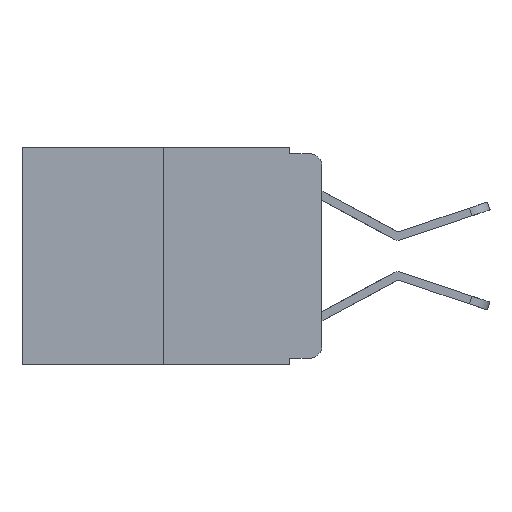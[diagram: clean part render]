
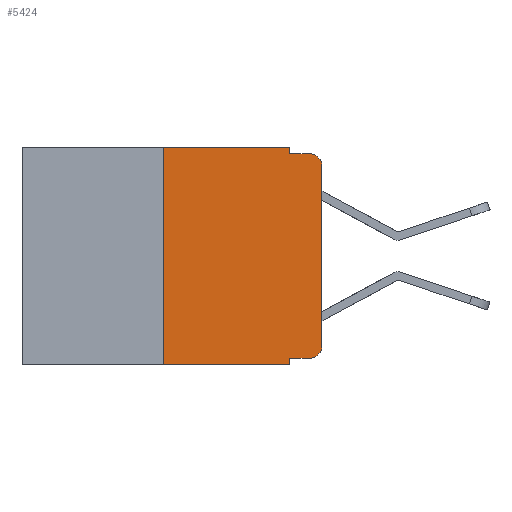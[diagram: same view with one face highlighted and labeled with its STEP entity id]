
A CAD part, left-side view. The second image highlights one B-rep face of the part: STEP entity #5424.
In plain terms, the highlighted planar face has unit normal (-1, 0, 0).
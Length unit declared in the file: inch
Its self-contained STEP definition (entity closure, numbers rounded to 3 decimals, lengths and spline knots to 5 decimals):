
#252 = CIRCLE ( 'NONE', #13759, 0.02 ) ;
#501 = DIRECTION ( 'NONE',  ( -1., 0., 0. ) ) ;
#651 = EDGE_LOOP ( 'NONE', ( #2425, #10456, #5234, #5033, #9141, #5659, #2915, #13785, #4641, #11686 ) ) ;
#1095 = PLANE ( 'NONE',  #2298 ) ;
#1150 = VERTEX_POINT ( 'NONE', #14654 ) ;
#1448 = DIRECTION ( 'NONE',  ( 0., 0., -1. ) ) ;
#1543 = EDGE_CURVE ( 'NONE', #1150, #5483, #14541, .T. ) ;
#2195 = EDGE_CURVE ( 'NONE', #3941, #1150, #7208, .T. ) ;
#2298 = AXIS2_PLACEMENT_3D ( 'NONE', #10191, #10025, #14856 ) ;
#2425 = ORIENTED_EDGE ( 'NONE', *, *, #8944, .T. ) ;
#2568 = CARTESIAN_POINT ( 'NONE',  ( 0., 0.051, -0.333 ) ) ;
#2664 = VERTEX_POINT ( 'NONE', #3519 ) ;
#2915 = ORIENTED_EDGE ( 'NONE', *, *, #10784, .T. ) ;
#3519 = CARTESIAN_POINT ( 'NONE',  ( 0., 0.051, -0.01 ) ) ;
#3877 = VECTOR ( 'NONE', #14405, 39.37008 ) ;
#3941 = VERTEX_POINT ( 'NONE', #12476 ) ;
#3961 = VECTOR ( 'NONE', #16169, 39.37008 ) ;
#4380 = LINE ( 'NONE', #8863, #3961 ) ;
#4381 = EDGE_CURVE ( 'NONE', #14129, #12838, #252, .T. ) ;
#4515 = DIRECTION ( 'NONE',  ( 0., 0., -1. ) ) ;
#4641 = ORIENTED_EDGE ( 'NONE', *, *, #7478, .T. ) ;
#4672 = VECTOR ( 'NONE', #12735, 39.37008 ) ;
#4751 = VERTEX_POINT ( 'NONE', #5886 ) ;
#4952 = EDGE_CURVE ( 'NONE', #13946, #15107, #12725, .T. ) ;
#5033 = ORIENTED_EDGE ( 'NONE', *, *, #6940, .F. ) ;
#5234 = ORIENTED_EDGE ( 'NONE', *, *, #15990, .F. ) ;
#5424 = ADVANCED_FACE ( 'NONE', ( #13089 ), #1095, .F. ) ;
#5483 = VERTEX_POINT ( 'NONE', #10083 ) ;
#5506 = CARTESIAN_POINT ( 'NONE',  ( 0., 0.02, -0.313 ) ) ;
#5659 = ORIENTED_EDGE ( 'NONE', *, *, #2195, .F. ) ;
#5664 = LINE ( 'NONE', #11074, #8600 ) ;
#5698 = VECTOR ( 'NONE', #11510, 39.37008 ) ;
#5886 = CARTESIAN_POINT ( 'NONE',  ( 0., 0.051, -0.343 ) ) ;
#6100 = DIRECTION ( 'NONE',  ( 0., 0., 1. ) ) ;
#6760 = DIRECTION ( 'NONE',  ( 0., 0., -1. ) ) ;
#6940 = EDGE_CURVE ( 'NONE', #5483, #2664, #12475, .T. ) ;
#6994 = CARTESIAN_POINT ( 'NONE',  ( 0., 0., -0.313 ) ) ;
#7208 = LINE ( 'NONE', #10082, #7602 ) ;
#7388 = VERTEX_POINT ( 'NONE', #12522 ) ;
#7478 = EDGE_CURVE ( 'NONE', #7388, #13946, #11147, .T. ) ;
#7602 = VECTOR ( 'NONE', #6100, 39.37008 ) ;
#7767 = VECTOR ( 'NONE', #10035, 39.37008 ) ;
#8401 = CARTESIAN_POINT ( 'NONE',  ( 0., 0.02, -0.03 ) ) ;
#8586 = DIRECTION ( 'NONE',  ( 0., -1., 0. ) ) ;
#8600 = VECTOR ( 'NONE', #8586, 39.37008 ) ;
#8863 = CARTESIAN_POINT ( 'NONE',  ( 0., 0.051, 0. ) ) ;
#8944 = EDGE_CURVE ( 'NONE', #15107, #14129, #10217, .T. ) ;
#9141 = ORIENTED_EDGE ( 'NONE', *, *, #1543, .F. ) ;
#9243 = CARTESIAN_POINT ( 'NONE',  ( 0., 0.051, 0. ) ) ;
#10025 = DIRECTION ( 'NONE',  ( 1., 0., 0. ) ) ;
#10035 = DIRECTION ( 'NONE',  ( 0., -1., 0. ) ) ;
#10082 = CARTESIAN_POINT ( 'NONE',  ( 0., 0.25, 0. ) ) ;
#10083 = CARTESIAN_POINT ( 'NONE',  ( 0., 0.051, 0. ) ) ;
#10191 = CARTESIAN_POINT ( 'NONE',  ( 0., 0.473, 0. ) ) ;
#10217 = LINE ( 'NONE', #10695, #3877 ) ;
#10456 = ORIENTED_EDGE ( 'NONE', *, *, #4381, .T. ) ;
#10690 = AXIS2_PLACEMENT_3D ( 'NONE', #5506, #14133, #6760 ) ;
#10695 = CARTESIAN_POINT ( 'NONE',  ( 0., 0., 0. ) ) ;
#10784 = EDGE_CURVE ( 'NONE', #3941, #4751, #5664, .T. ) ;
#11074 = CARTESIAN_POINT ( 'NONE',  ( 0., 0.473, -0.343 ) ) ;
#11147 = LINE ( 'NONE', #2568, #5698 ) ;
#11450 = LINE ( 'NONE', #13719, #7767 ) ;
#11510 = DIRECTION ( 'NONE',  ( 0., -1., 0. ) ) ;
#11516 = CARTESIAN_POINT ( 'NONE',  ( 0., 0.02, -0.01 ) ) ;
#11686 = ORIENTED_EDGE ( 'NONE', *, *, #4952, .T. ) ;
#12096 = VECTOR ( 'NONE', #1448, 39.37008 ) ;
#12475 = LINE ( 'NONE', #9243, #12096 ) ;
#12476 = CARTESIAN_POINT ( 'NONE',  ( 0., 0.25, -0.343 ) ) ;
#12522 = CARTESIAN_POINT ( 'NONE',  ( 0., 0.051, -0.333 ) ) ;
#12725 = CIRCLE ( 'NONE', #10690, 0.02 ) ;
#12735 = DIRECTION ( 'NONE',  ( 0., -1., 0. ) ) ;
#12753 = EDGE_CURVE ( 'NONE', #7388, #4751, #4380, .T. ) ;
#12838 = VERTEX_POINT ( 'NONE', #11516 ) ;
#13089 = FACE_OUTER_BOUND ( 'NONE', #651, .T. ) ;
#13719 = CARTESIAN_POINT ( 'NONE',  ( 0., 0.051, -0.01 ) ) ;
#13759 = AXIS2_PLACEMENT_3D ( 'NONE', #8401, #501, #4515 ) ;
#13785 = ORIENTED_EDGE ( 'NONE', *, *, #12753, .F. ) ;
#13946 = VERTEX_POINT ( 'NONE', #14234 ) ;
#14129 = VERTEX_POINT ( 'NONE', #15821 ) ;
#14133 = DIRECTION ( 'NONE',  ( -1., 0., 0. ) ) ;
#14234 = CARTESIAN_POINT ( 'NONE',  ( 0., 0.02, -0.333 ) ) ;
#14405 = DIRECTION ( 'NONE',  ( 0., 0., 1. ) ) ;
#14541 = LINE ( 'NONE', #15677, #4672 ) ;
#14654 = CARTESIAN_POINT ( 'NONE',  ( 0., 0.25, 0. ) ) ;
#14856 = DIRECTION ( 'NONE',  ( 0., 0., -1. ) ) ;
#15107 = VERTEX_POINT ( 'NONE', #6994 ) ;
#15677 = CARTESIAN_POINT ( 'NONE',  ( 0., 0.473, 0. ) ) ;
#15821 = CARTESIAN_POINT ( 'NONE',  ( 0., 0., -0.03 ) ) ;
#15990 = EDGE_CURVE ( 'NONE', #2664, #12838, #11450, .T. ) ;
#16169 = DIRECTION ( 'NONE',  ( 0., 0., -1. ) ) ;
